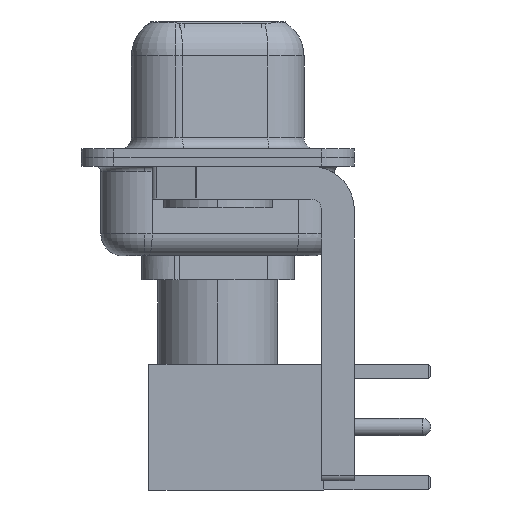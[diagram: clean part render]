
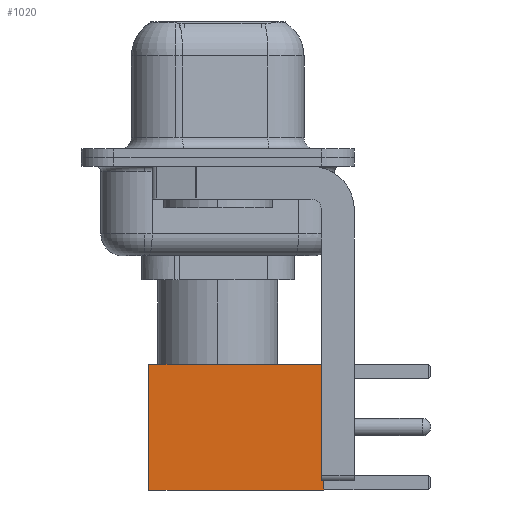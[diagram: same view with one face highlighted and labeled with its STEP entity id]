
A CAD part, left-side view. The second image highlights one B-rep face of the part: STEP entity #1020.
In plain terms, the highlighted face is planar.
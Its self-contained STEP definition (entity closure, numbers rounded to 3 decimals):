
#245 = EDGE_CURVE ( 'NONE', #7494, #4623, #16740, .T. ) ;
#494 = EDGE_CURVE ( 'NONE', #7494, #9016, #18684, .T. ) ;
#1020 = ADVANCED_FACE ( 'NONE', ( #17683 ), #11679, .T. ) ;
#1039 = CARTESIAN_POINT ( 'NONE',  ( 0., 2.875, 0. ) ) ;
#2293 = DIRECTION ( 'NONE',  ( -1., 0., 0. ) ) ;
#2301 = DIRECTION ( 'NONE',  ( 0., 0., -1. ) ) ;
#2618 = CARTESIAN_POINT ( 'NONE',  ( -2.875, 2.875, 0. ) ) ;
#3284 = DIRECTION ( 'NONE',  ( -1., 0., 0. ) ) ;
#3706 = CARTESIAN_POINT ( 'NONE',  ( 2.875, 2.875, 0. ) ) ;
#3845 = EDGE_CURVE ( 'NONE', #9016, #7544, #8310, .T. ) ;
#4623 = VERTEX_POINT ( 'NONE', #4974 ) ;
#4781 = LINE ( 'NONE', #6050, #19050 ) ;
#4974 = CARTESIAN_POINT ( 'NONE',  ( -2.875, 2.875, 8. ) ) ;
#6050 = CARTESIAN_POINT ( 'NONE',  ( -2.875, 2.875, 0. ) ) ;
#6075 = ORIENTED_EDGE ( 'NONE', *, *, #13841, .F. ) ;
#6749 = VECTOR ( 'NONE', #2301, 1000. ) ;
#7136 = CARTESIAN_POINT ( 'NONE',  ( 2.875, 2.875, 0. ) ) ;
#7494 = VERTEX_POINT ( 'NONE', #11435 ) ;
#7544 = VERTEX_POINT ( 'NONE', #2618 ) ;
#8310 = LINE ( 'NONE', #1039, #16370 ) ;
#8320 = CARTESIAN_POINT ( 'NONE',  ( 2.875, 2.875, 0. ) ) ;
#9016 = VERTEX_POINT ( 'NONE', #3706 ) ;
#9196 = EDGE_LOOP ( 'NONE', ( #10862, #14031, #6075, #9778 ) ) ;
#9234 = DIRECTION ( 'NONE',  ( 0., 0., -1. ) ) ;
#9778 = ORIENTED_EDGE ( 'NONE', *, *, #245, .F. ) ;
#10126 = DIRECTION ( 'NONE',  ( 0., 0., 1. ) ) ;
#10862 = ORIENTED_EDGE ( 'NONE', *, *, #494, .T. ) ;
#11306 = AXIS2_PLACEMENT_3D ( 'NONE', #7136, #16123, #10126 ) ;
#11435 = CARTESIAN_POINT ( 'NONE',  ( 2.875, 2.875, 8. ) ) ;
#11679 = PLANE ( 'NONE',  #11306 ) ;
#12016 = VECTOR ( 'NONE', #3284, 1000. ) ;
#13729 = CARTESIAN_POINT ( 'NONE',  ( 0., 2.875, 8. ) ) ;
#13841 = EDGE_CURVE ( 'NONE', #4623, #7544, #4781, .T. ) ;
#14031 = ORIENTED_EDGE ( 'NONE', *, *, #3845, .T. ) ;
#16123 = DIRECTION ( 'NONE',  ( 0., 1., 0. ) ) ;
#16370 = VECTOR ( 'NONE', #2293, 1000. ) ;
#16740 = LINE ( 'NONE', #13729, #12016 ) ;
#17683 = FACE_OUTER_BOUND ( 'NONE', #9196, .T. ) ;
#18684 = LINE ( 'NONE', #8320, #6749 ) ;
#19050 = VECTOR ( 'NONE', #9234, 1000. ) ;
